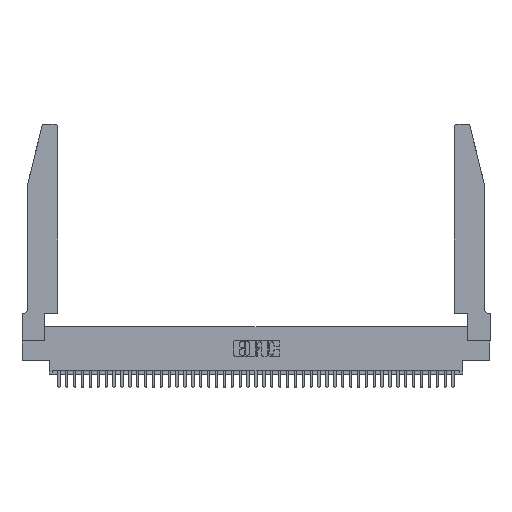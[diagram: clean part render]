
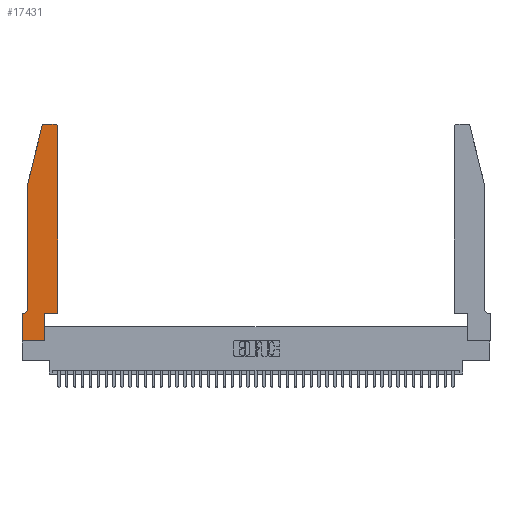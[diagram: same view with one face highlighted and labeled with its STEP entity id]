
A CAD part, top view. The second image highlights one B-rep face of the part: STEP entity #17431.
In plain terms, the highlighted planar face has unit normal (0, 0, 1).
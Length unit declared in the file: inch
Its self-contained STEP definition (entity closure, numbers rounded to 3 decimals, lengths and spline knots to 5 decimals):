
#129 = VERTEX_POINT ( 'NONE', #22738 ) ;
#1508 = DIRECTION ( 'NONE',  ( 0., -1., 0. ) ) ;
#1870 = EDGE_CURVE ( 'NONE', #29553, #21554, #5493, .T. ) ;
#2399 = DIRECTION ( 'NONE',  ( 0., 0., -1. ) ) ;
#3278 = AXIS2_PLACEMENT_3D ( 'NONE', #14812, #38466, #41847 ) ;
#3388 = VECTOR ( 'NONE', #7044, 39.37008 ) ;
#4085 = EDGE_CURVE ( 'NONE', #23902, #28014, #20766, .T. ) ;
#4107 = VERTEX_POINT ( 'NONE', #4900 ) ;
#4303 = CARTESIAN_POINT ( 'NONE',  ( 0.4505, 0.35, 0.37 ) ) ;
#4772 = FACE_OUTER_BOUND ( 'NONE', #10451, .T. ) ;
#4900 = CARTESIAN_POINT ( 'NONE',  ( 0.4205, 2.75, 0.37 ) ) ;
#5047 = CARTESIAN_POINT ( 'NONE',  ( 0.0055, 0.42, 0.37 ) ) ;
#5322 = VECTOR ( 'NONE', #23298, 39.37008 ) ;
#5389 = DIRECTION ( 'NONE',  ( 0., 1., 0. ) ) ;
#5493 = LINE ( 'NONE', #35011, #27194 ) ;
#5881 = AXIS2_PLACEMENT_3D ( 'NONE', #23024, #26699, #33545 ) ;
#6169 = EDGE_CURVE ( 'NONE', #43007, #42653, #22121, .T. ) ;
#6443 = LINE ( 'NONE', #42244, #41382 ) ;
#6712 = VECTOR ( 'NONE', #1508, 39.37008 ) ;
#7044 = DIRECTION ( 'NONE',  ( -0.239, -0.971, 0. ) ) ;
#8197 = VERTEX_POINT ( 'NONE', #27436 ) ;
#8373 = CARTESIAN_POINT ( 'NONE',  ( 0.0755, 2., 0.37 ) ) ;
#9301 = DIRECTION ( 'NONE',  ( 1., 0., 0. ) ) ;
#9583 = CARTESIAN_POINT ( 'NONE',  ( 0.0755, 0.35, 0.37 ) ) ;
#10185 = VECTOR ( 'NONE', #29542, 39.37008 ) ;
#10275 = ORIENTED_EDGE ( 'NONE', *, *, #4085, .T. ) ;
#10451 = EDGE_LOOP ( 'NONE', ( #30843, #11725, #26469, #35957, #10275, #27653, #36413, #41274, #42530, #23330, #19315, #25727 ) ) ;
#10713 = AXIS2_PLACEMENT_3D ( 'NONE', #10734, #17524, #37790 ) ;
#10734 = CARTESIAN_POINT ( 'NONE',  ( 0., 0.35, 0.37 ) ) ;
#11725 = ORIENTED_EDGE ( 'NONE', *, *, #6169, .T. ) ;
#12252 = LINE ( 'NONE', #8373, #6712 ) ;
#12367 = EDGE_CURVE ( 'NONE', #28014, #31156, #41910, .T. ) ;
#12854 = DIRECTION ( 'NONE',  ( 0., -1., 0. ) ) ;
#12941 = EDGE_CURVE ( 'NONE', #15666, #23902, #12252, .T. ) ;
#13098 = CIRCLE ( 'NONE', #3278, 0.03 ) ;
#13319 = LINE ( 'NONE', #19902, #5322 ) ;
#13367 = LINE ( 'NONE', #32669, #19170 ) ;
#14366 = CARTESIAN_POINT ( 'NONE',  ( 0., 0.35, 0.37 ) ) ;
#14812 = CARTESIAN_POINT ( 'NONE',  ( 0.4205, 2.72, 0.37 ) ) ;
#15329 = CARTESIAN_POINT ( 'NONE',  ( 0.284, 2.75, 0.37 ) ) ;
#15666 = VERTEX_POINT ( 'NONE', #24113 ) ;
#15842 = EDGE_CURVE ( 'NONE', #8197, #4107, #13098, .T. ) ;
#16993 = EDGE_CURVE ( 'NONE', #29248, #8197, #6443, .T. ) ;
#17121 = EDGE_CURVE ( 'NONE', #4107, #43007, #13319, .T. ) ;
#17431 = ADVANCED_FACE ( 'NONE', ( #4772 ), #17955, .T. ) ;
#17524 = DIRECTION ( 'NONE',  ( 0., 0., 1. ) ) ;
#17955 = PLANE ( 'NONE',  #10713 ) ;
#18169 = CARTESIAN_POINT ( 'NONE',  ( 0.2865, 0., 0.37 ) ) ;
#18264 = DIRECTION ( 'NONE',  ( 0., 1., 0. ) ) ;
#18317 = CARTESIAN_POINT ( 'NONE',  ( 0.0755, 0.42, 0.37 ) ) ;
#19170 = VECTOR ( 'NONE', #12854, 39.37008 ) ;
#19315 = ORIENTED_EDGE ( 'NONE', *, *, #16993, .T. ) ;
#19533 = LINE ( 'NONE', #25848, #38012 ) ;
#19902 = CARTESIAN_POINT ( 'NONE',  ( 0.2605, 2.75, 0.37 ) ) ;
#20766 = CIRCLE ( 'NONE', #22303, 0.07 ) ;
#21554 = VERTEX_POINT ( 'NONE', #32750 ) ;
#22121 = CIRCLE ( 'NONE', #5881, 0.03 ) ;
#22303 = AXIS2_PLACEMENT_3D ( 'NONE', #5047, #2399, #39695 ) ;
#22738 = CARTESIAN_POINT ( 'NONE',  ( 0., 0., 0.37 ) ) ;
#23024 = CARTESIAN_POINT ( 'NONE',  ( 0.284, 2.72, 0.37 ) ) ;
#23298 = DIRECTION ( 'NONE',  ( -1., 0., 0. ) ) ;
#23330 = ORIENTED_EDGE ( 'NONE', *, *, #37610, .T. ) ;
#23879 = LINE ( 'NONE', #4303, #30787 ) ;
#23902 = VERTEX_POINT ( 'NONE', #18317 ) ;
#24113 = CARTESIAN_POINT ( 'NONE',  ( 0.0755, 2., 0.37 ) ) ;
#25727 = ORIENTED_EDGE ( 'NONE', *, *, #15842, .T. ) ;
#25848 = CARTESIAN_POINT ( 'NONE',  ( 0., 0., 0.37 ) ) ;
#26469 = ORIENTED_EDGE ( 'NONE', *, *, #42637, .T. ) ;
#26699 = DIRECTION ( 'NONE',  ( 0., 0., 1. ) ) ;
#27194 = VECTOR ( 'NONE', #18264, 39.37008 ) ;
#27436 = CARTESIAN_POINT ( 'NONE',  ( 0.4505, 2.72, 0.37 ) ) ;
#27653 = ORIENTED_EDGE ( 'NONE', *, *, #12367, .T. ) ;
#28014 = VERTEX_POINT ( 'NONE', #31019 ) ;
#29248 = VERTEX_POINT ( 'NONE', #40379 ) ;
#29542 = DIRECTION ( 'NONE',  ( -1., 0., 0. ) ) ;
#29553 = VERTEX_POINT ( 'NONE', #18169 ) ;
#29718 = EDGE_CURVE ( 'NONE', #129, #29553, #19533, .T. ) ;
#30409 = LINE ( 'NONE', #33564, #3388 ) ;
#30787 = VECTOR ( 'NONE', #38079, 39.37008 ) ;
#30843 = ORIENTED_EDGE ( 'NONE', *, *, #17121, .T. ) ;
#31019 = CARTESIAN_POINT ( 'NONE',  ( 0.0055, 0.35, 0.37 ) ) ;
#31156 = VERTEX_POINT ( 'NONE', #14366 ) ;
#32669 = CARTESIAN_POINT ( 'NONE',  ( 0., 0., 0.37 ) ) ;
#32750 = CARTESIAN_POINT ( 'NONE',  ( 0.2865, 0.35, 0.37 ) ) ;
#33545 = DIRECTION ( 'NONE',  ( 1., 0., 0. ) ) ;
#33564 = CARTESIAN_POINT ( 'NONE',  ( 0.0755, 2., 0.37 ) ) ;
#35011 = CARTESIAN_POINT ( 'NONE',  ( 0.2865, 0.35, 0.37 ) ) ;
#35957 = ORIENTED_EDGE ( 'NONE', *, *, #12941, .T. ) ;
#36413 = ORIENTED_EDGE ( 'NONE', *, *, #38380, .T. ) ;
#37610 = EDGE_CURVE ( 'NONE', #21554, #29248, #23879, .T. ) ;
#37790 = DIRECTION ( 'NONE',  ( 1., 0., 0. ) ) ;
#38012 = VECTOR ( 'NONE', #9301, 39.37008 ) ;
#38079 = DIRECTION ( 'NONE',  ( 1., 0., 0. ) ) ;
#38380 = EDGE_CURVE ( 'NONE', #31156, #129, #13367, .T. ) ;
#38466 = DIRECTION ( 'NONE',  ( 0., 0., 1. ) ) ;
#39695 = DIRECTION ( 'NONE',  ( -1., 0., 0. ) ) ;
#40334 = CARTESIAN_POINT ( 'NONE',  ( 0.25487, 2.72718, 0.37 ) ) ;
#40379 = CARTESIAN_POINT ( 'NONE',  ( 0.4505, 0.35, 0.37 ) ) ;
#41274 = ORIENTED_EDGE ( 'NONE', *, *, #29718, .T. ) ;
#41382 = VECTOR ( 'NONE', #5389, 39.37008 ) ;
#41847 = DIRECTION ( 'NONE',  ( 1., 0., 0. ) ) ;
#41910 = LINE ( 'NONE', #9583, #10185 ) ;
#42244 = CARTESIAN_POINT ( 'NONE',  ( 0.4505, 0.35, 0.37 ) ) ;
#42530 = ORIENTED_EDGE ( 'NONE', *, *, #1870, .T. ) ;
#42637 = EDGE_CURVE ( 'NONE', #42653, #15666, #30409, .T. ) ;
#42653 = VERTEX_POINT ( 'NONE', #40334 ) ;
#43007 = VERTEX_POINT ( 'NONE', #15329 ) ;
